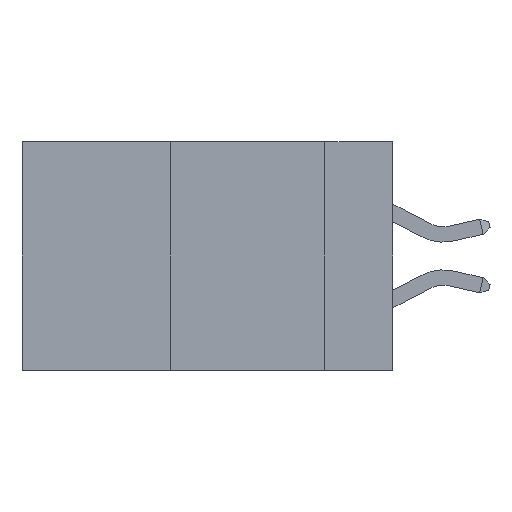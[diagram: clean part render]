
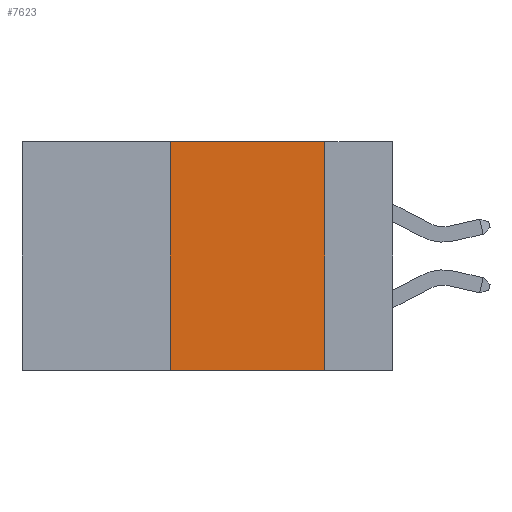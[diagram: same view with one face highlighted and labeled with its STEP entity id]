
A CAD part, left-side view. The second image highlights one B-rep face of the part: STEP entity #7623.
In plain terms, the highlighted planar face has unit normal (-1, 0, 0).
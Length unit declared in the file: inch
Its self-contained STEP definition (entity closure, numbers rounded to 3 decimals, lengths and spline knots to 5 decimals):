
#1400 = AXIS2_PLACEMENT_3D ( 'NONE', #12362, #11257, #7700 ) ;
#1537 = FACE_OUTER_BOUND ( 'NONE', #12905, .T. ) ;
#1889 = VECTOR ( 'NONE', #4157, 39.37008 ) ;
#2416 = CARTESIAN_POINT ( 'NONE',  ( 0., 0.6, -0.37 ) ) ;
#2582 = ORIENTED_EDGE ( 'NONE', *, *, #14175, .F. ) ;
#3033 = EDGE_CURVE ( 'NONE', #12331, #9667, #7805, .T. ) ;
#3415 = DIRECTION ( 'NONE',  ( 0., -1., 0. ) ) ;
#4157 = DIRECTION ( 'NONE',  ( 0., 0., -1. ) ) ;
#4196 = CARTESIAN_POINT ( 'NONE',  ( 0., 0.11, 0. ) ) ;
#4266 = ORIENTED_EDGE ( 'NONE', *, *, #3033, .F. ) ;
#4491 = EDGE_CURVE ( 'NONE', #12331, #8587, #5581, .T. ) ;
#5373 = ORIENTED_EDGE ( 'NONE', *, *, #4491, .T. ) ;
#5581 = LINE ( 'NONE', #2416, #14839 ) ;
#6302 = VECTOR ( 'NONE', #11680, 39.37008 ) ;
#7623 = ADVANCED_FACE ( 'NONE', ( #1537 ), #7752, .F. ) ;
#7700 = DIRECTION ( 'NONE',  ( 0., 0., -1. ) ) ;
#7752 = PLANE ( 'NONE',  #1400 ) ;
#7805 = LINE ( 'NONE', #7814, #10725 ) ;
#7814 = CARTESIAN_POINT ( 'NONE',  ( 0., 0.36, 0. ) ) ;
#8587 = VERTEX_POINT ( 'NONE', #12302 ) ;
#9667 = VERTEX_POINT ( 'NONE', #12581 ) ;
#9830 = EDGE_CURVE ( 'NONE', #13390, #8587, #10961, .T. ) ;
#10062 = DIRECTION ( 'NONE',  ( 0., 0., 1. ) ) ;
#10569 = CARTESIAN_POINT ( 'NONE',  ( 0., 0.6, 0. ) ) ;
#10725 = VECTOR ( 'NONE', #10062, 39.37008 ) ;
#10961 = LINE ( 'NONE', #14514, #1889 ) ;
#11257 = DIRECTION ( 'NONE',  ( 1., 0., 0. ) ) ;
#11680 = DIRECTION ( 'NONE',  ( 0., -1., 0. ) ) ;
#12134 = CARTESIAN_POINT ( 'NONE',  ( 0., 0.36, -0.37 ) ) ;
#12302 = CARTESIAN_POINT ( 'NONE',  ( 0., 0.11, -0.37 ) ) ;
#12331 = VERTEX_POINT ( 'NONE', #12134 ) ;
#12362 = CARTESIAN_POINT ( 'NONE',  ( 0., 0.6, 0. ) ) ;
#12581 = CARTESIAN_POINT ( 'NONE',  ( 0., 0.36, 0. ) ) ;
#12905 = EDGE_LOOP ( 'NONE', ( #14965, #2582, #4266, #5373 ) ) ;
#13390 = VERTEX_POINT ( 'NONE', #4196 ) ;
#13907 = LINE ( 'NONE', #10569, #6302 ) ;
#14175 = EDGE_CURVE ( 'NONE', #9667, #13390, #13907, .T. ) ;
#14514 = CARTESIAN_POINT ( 'NONE',  ( 0., 0.11, 0. ) ) ;
#14839 = VECTOR ( 'NONE', #3415, 39.37008 ) ;
#14965 = ORIENTED_EDGE ( 'NONE', *, *, #9830, .F. ) ;
